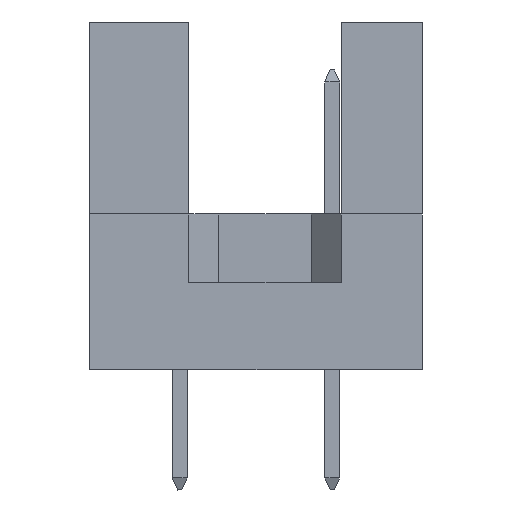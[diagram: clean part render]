
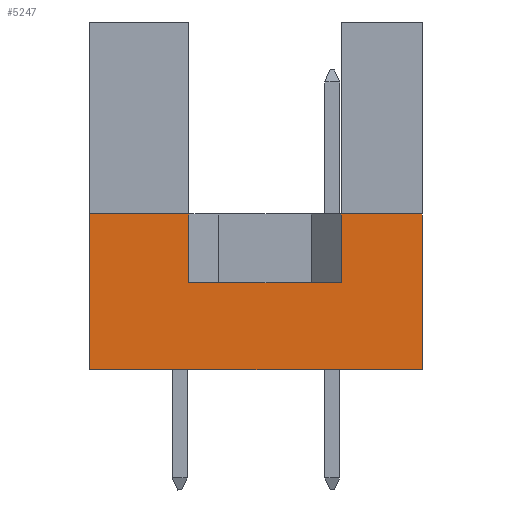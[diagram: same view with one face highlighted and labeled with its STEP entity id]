
A CAD part, left-side view. The second image highlights one B-rep face of the part: STEP entity #5247.
In plain terms, the highlighted planar face has unit normal (-1, 0, 0).
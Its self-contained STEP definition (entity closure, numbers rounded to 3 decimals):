
#215 = AXIS2_PLACEMENT_3D ( 'NONE', #8416, #4474, #6115 ) ;
#241 = CARTESIAN_POINT ( 'NONE',  ( -27.5, 0., 5.2 ) ) ;
#660 = LINE ( 'NONE', #7607, #7386 ) ;
#689 = VECTOR ( 'NONE', #4215, 1000. ) ;
#805 = PLANE ( 'NONE',  #215 ) ;
#1450 = FACE_OUTER_BOUND ( 'NONE', #8840, .T. ) ;
#1455 = ORIENTED_EDGE ( 'NONE', *, *, #5526, .T. ) ;
#1480 = CARTESIAN_POINT ( 'NONE',  ( -27.5, 7.79, 2.9 ) ) ;
#1502 = VECTOR ( 'NONE', #4513, 1000. ) ;
#1735 = CARTESIAN_POINT ( 'NONE',  ( -27.5, 7.79, 2.9 ) ) ;
#1741 = DIRECTION ( 'NONE',  ( 0., -1., 0. ) ) ;
#1747 = VERTEX_POINT ( 'NONE', #4331 ) ;
#2255 = CARTESIAN_POINT ( 'NONE',  ( -27.5, 2.71, 2.9 ) ) ;
#2298 = VERTEX_POINT ( 'NONE', #7414 ) ;
#2537 = EDGE_CURVE ( 'NONE', #2298, #3528, #8567, .T. ) ;
#2698 = VECTOR ( 'NONE', #1741, 1000. ) ;
#2810 = ORIENTED_EDGE ( 'NONE', *, *, #5398, .F. ) ;
#3251 = LINE ( 'NONE', #7675, #4514 ) ;
#3528 = VERTEX_POINT ( 'NONE', #5576 ) ;
#3700 = CARTESIAN_POINT ( 'NONE',  ( -27.5, 11.1, 5.2 ) ) ;
#4199 = VERTEX_POINT ( 'NONE', #4308 ) ;
#4215 = DIRECTION ( 'NONE',  ( 0., 0., 1. ) ) ;
#4228 = CARTESIAN_POINT ( 'NONE',  ( -27.5, 2.71, 5.2 ) ) ;
#4308 = CARTESIAN_POINT ( 'NONE',  ( -27.5, 11.1, 5.2 ) ) ;
#4331 = CARTESIAN_POINT ( 'NONE',  ( -27.5, 7.79, 5.2 ) ) ;
#4350 = EDGE_CURVE ( 'NONE', #9080, #8662, #9202, .T. ) ;
#4474 = DIRECTION ( 'NONE',  ( 1., 0., 0. ) ) ;
#4478 = VERTEX_POINT ( 'NONE', #241 ) ;
#4513 = DIRECTION ( 'NONE',  ( 0., -1., 0. ) ) ;
#4514 = VECTOR ( 'NONE', #6951, 1000. ) ;
#4572 = ORIENTED_EDGE ( 'NONE', *, *, #5212, .F. ) ;
#5057 = VERTEX_POINT ( 'NONE', #4228 ) ;
#5063 = DIRECTION ( 'NONE',  ( 0., 0., 1. ) ) ;
#5107 = ORIENTED_EDGE ( 'NONE', *, *, #2537, .T. ) ;
#5206 = DIRECTION ( 'NONE',  ( 0., -1., 0. ) ) ;
#5212 = EDGE_CURVE ( 'NONE', #4199, #1747, #660, .T. ) ;
#5229 = ORIENTED_EDGE ( 'NONE', *, *, #9508, .F. ) ;
#5247 = ADVANCED_FACE ( 'NONE', ( #1450 ), #805, .F. ) ;
#5398 = EDGE_CURVE ( 'NONE', #2298, #4199, #8905, .T. ) ;
#5480 = VECTOR ( 'NONE', #5206, 1000. ) ;
#5526 = EDGE_CURVE ( 'NONE', #9080, #1747, #5670, .T. ) ;
#5576 = CARTESIAN_POINT ( 'NONE',  ( -27.5, 0., 0. ) ) ;
#5618 = VECTOR ( 'NONE', #8333, 1000. ) ;
#5670 = LINE ( 'NONE', #8861, #6249 ) ;
#6115 = DIRECTION ( 'NONE',  ( 0., 0., -1. ) ) ;
#6249 = VECTOR ( 'NONE', #5063, 1000. ) ;
#6471 = CARTESIAN_POINT ( 'NONE',  ( -27.5, 11.1, 0. ) ) ;
#6650 = LINE ( 'NONE', #2255, #5618 ) ;
#6951 = DIRECTION ( 'NONE',  ( 0., 0., 1. ) ) ;
#7075 = ORIENTED_EDGE ( 'NONE', *, *, #4350, .F. ) ;
#7386 = VECTOR ( 'NONE', #9018, 1000. ) ;
#7414 = CARTESIAN_POINT ( 'NONE',  ( -27.5, 11.1, 0. ) ) ;
#7450 = EDGE_CURVE ( 'NONE', #5057, #4478, #8295, .T. ) ;
#7607 = CARTESIAN_POINT ( 'NONE',  ( -27.5, 11.1, 5.2 ) ) ;
#7675 = CARTESIAN_POINT ( 'NONE',  ( -27.5, 0., 0. ) ) ;
#7964 = CARTESIAN_POINT ( 'NONE',  ( -27.5, 2.71, 2.9 ) ) ;
#8035 = ORIENTED_EDGE ( 'NONE', *, *, #9657, .T. ) ;
#8295 = LINE ( 'NONE', #3700, #5480 ) ;
#8333 = DIRECTION ( 'NONE',  ( 0., 0., 1. ) ) ;
#8416 = CARTESIAN_POINT ( 'NONE',  ( -27.5, 11.1, 0. ) ) ;
#8567 = LINE ( 'NONE', #9597, #2698 ) ;
#8662 = VERTEX_POINT ( 'NONE', #7964 ) ;
#8840 = EDGE_LOOP ( 'NONE', ( #7075, #1455, #4572, #2810, #5107, #8035, #8871, #5229 ) ) ;
#8861 = CARTESIAN_POINT ( 'NONE',  ( -27.5, 7.79, 2.9 ) ) ;
#8871 = ORIENTED_EDGE ( 'NONE', *, *, #7450, .F. ) ;
#8905 = LINE ( 'NONE', #6471, #689 ) ;
#9018 = DIRECTION ( 'NONE',  ( 0., -1., 0. ) ) ;
#9080 = VERTEX_POINT ( 'NONE', #1735 ) ;
#9202 = LINE ( 'NONE', #1480, #1502 ) ;
#9508 = EDGE_CURVE ( 'NONE', #8662, #5057, #6650, .T. ) ;
#9597 = CARTESIAN_POINT ( 'NONE',  ( -27.5, 11.1, 0. ) ) ;
#9657 = EDGE_CURVE ( 'NONE', #3528, #4478, #3251, .T. ) ;
